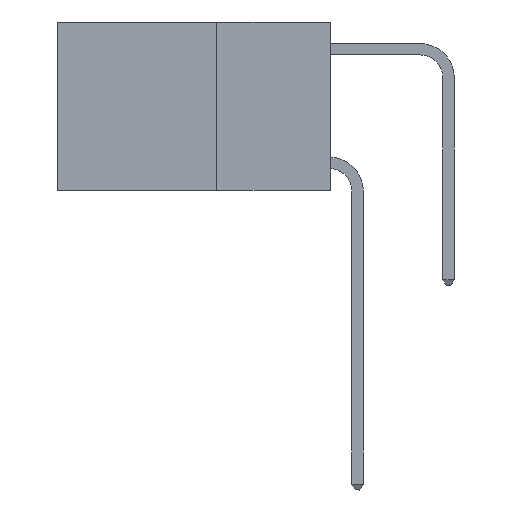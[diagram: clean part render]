
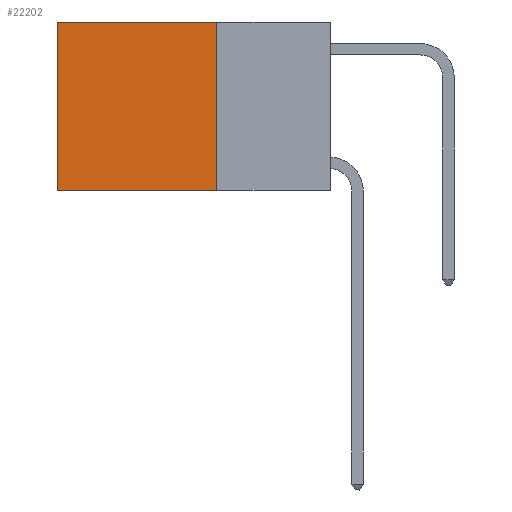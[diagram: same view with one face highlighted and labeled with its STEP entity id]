
A CAD part, left-side view. The second image highlights one B-rep face of the part: STEP entity #22202.
In plain terms, the highlighted planar face has unit normal (-1, 0, 0).
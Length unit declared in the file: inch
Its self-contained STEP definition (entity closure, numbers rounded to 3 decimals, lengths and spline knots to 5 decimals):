
#1884 = CARTESIAN_POINT ( 'NONE',  ( 0.2625, 0.25, -0.37 ) ) ;
#1961 = CARTESIAN_POINT ( 'NONE',  ( 0.2625, 0.6, 0. ) ) ;
#2507 = DIRECTION ( 'NONE',  ( 0., 0., -1. ) ) ;
#3021 = VECTOR ( 'NONE', #4822, 39.37008 ) ;
#3042 = CARTESIAN_POINT ( 'NONE',  ( 0.2625, 0.6, 0. ) ) ;
#3456 = CARTESIAN_POINT ( 'NONE',  ( 0.2625, 0.25, 0. ) ) ;
#4209 = EDGE_CURVE ( 'NONE', #15111, #18081, #4563, .T. ) ;
#4563 = LINE ( 'NONE', #24149, #13110 ) ;
#4819 = ORIENTED_EDGE ( 'NONE', *, *, #26918, .F. ) ;
#4822 = DIRECTION ( 'NONE',  ( 0., 0., -1. ) ) ;
#6303 = LINE ( 'NONE', #3456, #16158 ) ;
#7732 = ORIENTED_EDGE ( 'NONE', *, *, #4209, .F. ) ;
#13110 = VECTOR ( 'NONE', #2507, 39.37008 ) ;
#13335 = CARTESIAN_POINT ( 'NONE',  ( 0.2625, 0.25, -0.37 ) ) ;
#13526 = AXIS2_PLACEMENT_3D ( 'NONE', #17595, #17443, #27081 ) ;
#14638 = ORIENTED_EDGE ( 'NONE', *, *, #28573, .T. ) ;
#15111 = VERTEX_POINT ( 'NONE', #30811 ) ;
#16158 = VECTOR ( 'NONE', #27315, 39.37008 ) ;
#16427 = LINE ( 'NONE', #1884, #18193 ) ;
#17118 = FACE_OUTER_BOUND ( 'NONE', #17770, .T. ) ;
#17151 = VERTEX_POINT ( 'NONE', #3042 ) ;
#17443 = DIRECTION ( 'NONE',  ( 1., 0., 0. ) ) ;
#17595 = CARTESIAN_POINT ( 'NONE',  ( 0.2625, 0.25, 0. ) ) ;
#17770 = EDGE_LOOP ( 'NONE', ( #19216, #4819, #7732, #14638 ) ) ;
#18081 = VERTEX_POINT ( 'NONE', #13335 ) ;
#18193 = VECTOR ( 'NONE', #21001, 39.37008 ) ;
#19216 = ORIENTED_EDGE ( 'NONE', *, *, #27374, .T. ) ;
#21001 = DIRECTION ( 'NONE',  ( 0., 1., 0. ) ) ;
#21481 = VERTEX_POINT ( 'NONE', #23800 ) ;
#22202 = ADVANCED_FACE ( 'NONE', ( #17118 ), #26761, .F. ) ;
#23800 = CARTESIAN_POINT ( 'NONE',  ( 0.2625, 0.6, -0.37 ) ) ;
#24149 = CARTESIAN_POINT ( 'NONE',  ( 0.2625, 0.25, 0. ) ) ;
#26761 = PLANE ( 'NONE',  #13526 ) ;
#26918 = EDGE_CURVE ( 'NONE', #18081, #21481, #16427, .T. ) ;
#27081 = DIRECTION ( 'NONE',  ( 0., 0., -1. ) ) ;
#27315 = DIRECTION ( 'NONE',  ( 0., 1., 0. ) ) ;
#27374 = EDGE_CURVE ( 'NONE', #17151, #21481, #30873, .T. ) ;
#28573 = EDGE_CURVE ( 'NONE', #15111, #17151, #6303, .T. ) ;
#30811 = CARTESIAN_POINT ( 'NONE',  ( 0.2625, 0.25, 0. ) ) ;
#30873 = LINE ( 'NONE', #1961, #3021 ) ;
